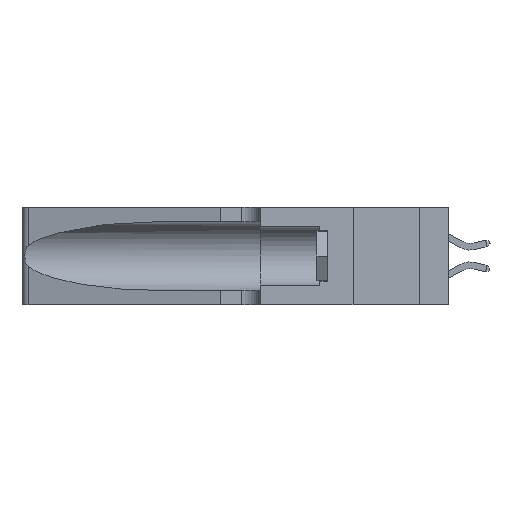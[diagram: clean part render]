
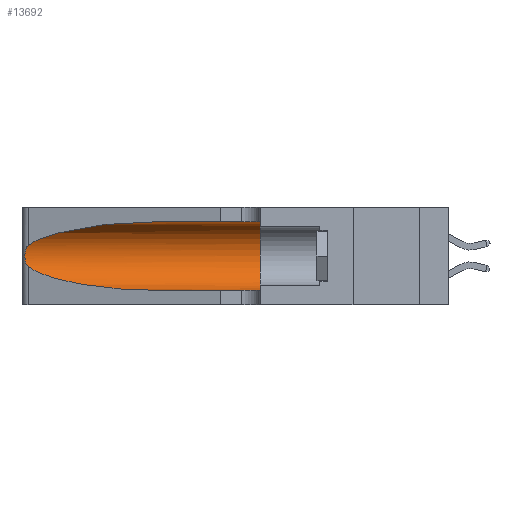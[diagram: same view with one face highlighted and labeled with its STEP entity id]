
A CAD part, left-side view. The second image highlights one B-rep face of the part: STEP entity #13692.
In plain terms, the highlighted cylindrical face has radius 3.308 mm (diameter 6.617 mm), a partial arc.
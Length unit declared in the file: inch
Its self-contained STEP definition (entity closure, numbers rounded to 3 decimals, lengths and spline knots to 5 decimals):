
#165 = FACE_OUTER_BOUND ( 'NONE', #13969, .T. ) ;
#880 = CARTESIAN_POINT ( 'NONE',  ( 0.1305, 0.72297, 0.05475 ) ) ;
#1026 = CARTESIAN_POINT ( 'NONE',  ( 0.25856, 1.23593, 0.16098 ) ) ;
#2822 = CARTESIAN_POINT ( 'NONE',  ( 0.1305, 1.61858, 0.05475 ) ) ;
#2941 = CARTESIAN_POINT ( 'NONE',  ( 0.25787, 1.23484, 0.2124 ) ) ;
#3270 = EDGE_CURVE ( 'NONE', #7609, #3434, #14867, .T. ) ;
#3434 = VERTEX_POINT ( 'NONE', #4056 ) ;
#3555 = LINE ( 'NONE', #2822, #7348 ) ;
#3957 = ORIENTED_EDGE ( 'NONE', *, *, #7733, .F. ) ;
#4056 = CARTESIAN_POINT ( 'NONE',  ( 0.25487, 1.22718, 0.22369 ) ) ;
#4150 = B_SPLINE_CURVE_WITH_KNOTS ( 'NONE', 3,
 ( #14996, #6433, #4385, #2941, #21763, #4460, #9766, #11475, #15070, #1026, #11397, #13163, #4609, #7867 ),
 .UNSPECIFIED., .F., .F.,
 ( 4, 2, 2, 2, 2, 2, 4 ),
 ( 0., 0.00027, 0.00053, 0.00107, 0.0016, 0.00187, 0.00214 ),
 .UNSPECIFIED. ) ;
#4385 = CARTESIAN_POINT ( 'NONE',  ( 0.25639, 1.23184, 0.21858 ) ) ;
#4460 = CARTESIAN_POINT ( 'NONE',  ( 0.26018, 1.23835, 0.19895 ) ) ;
#4533 = CARTESIAN_POINT ( 'NONE',  ( 0.1305, 0.72297, 0.31525 ) ) ;
#4609 = CARTESIAN_POINT ( 'NONE',  ( 0.25555, 1.22993, 0.14849 ) ) ;
#4737 = CARTESIAN_POINT ( 'NONE',  ( 0.25487, 1.22718, 0.22369 ) ) ;
#5417 = DIRECTION ( 'NONE',  ( 0., 1., 0. ) ) ;
#5689 = CARTESIAN_POINT ( 'NONE',  ( 0.1305, 1.61858, 0.31525 ) ) ;
#6272 = CARTESIAN_POINT ( 'NONE',  ( 0.1305, 0.72297, 0.31525 ) ) ;
#6433 = CARTESIAN_POINT ( 'NONE',  ( 0.25555, 1.22994, 0.2215 ) ) ;
#6752 = ORIENTED_EDGE ( 'NONE', *, *, #13815, .F. ) ;
#6821 = CARTESIAN_POINT ( 'NONE',  ( 0.1305, 0.35, 0.31525 ) ) ;
#7101 = CARTESIAN_POINT ( 'NONE',  ( 0.25487, 1.22718, 0.14631 ) ) ;
#7280 = VERTEX_POINT ( 'NONE', #6821 ) ;
#7348 = VECTOR ( 'NONE', #20287, 39.37008 ) ;
#7609 = VERTEX_POINT ( 'NONE', #4533 ) ;
#7733 = EDGE_CURVE ( 'NONE', #7280, #18139, #19593, .T. ) ;
#7867 = CARTESIAN_POINT ( 'NONE',  ( 0.25487, 1.22718, 0.14631 ) ) ;
#8226 = CARTESIAN_POINT ( 'NONE',  ( 0.2373, 1.15595, 0.28018 ) ) ;
#9071 = AXIS2_PLACEMENT_3D ( 'NONE', #10412, #5417, #20990 ) ;
#9357 = ORIENTED_EDGE ( 'NONE', *, *, #20244, .T. ) ;
#9373 = CARTESIAN_POINT ( 'NONE',  ( 0.25487, 1.22718, 0.14631 ) ) ;
#9447 = CARTESIAN_POINT ( 'NONE',  ( 0.1305, 0.72297, 0.05475 ) ) ;
#9766 = CARTESIAN_POINT ( 'NONE',  ( 0.26075, 1.23896, 0.19203 ) ) ;
#9852 =( BOUNDED_CURVE ( )  B_SPLINE_CURVE ( 3, ( #9373, #21517, #12824, #9447 ),
 .UNSPECIFIED., .F., .F. ) 
 B_SPLINE_CURVE_WITH_KNOTS ( ( 4, 4 ),
 ( 3.44316, 4.71239 ),
 .UNSPECIFIED. ) 
 CURVE ( )  GEOMETRIC_REPRESENTATION_ITEM ( )  RATIONAL_B_SPLINE_CURVE ( ( 1., 0.87, 0.87, 1. ) ) 
 REPRESENTATION_ITEM ( '' )  );
#9864 = AXIS2_PLACEMENT_3D ( 'NONE', #13708, #13776, #15459 ) ;
#10412 = CARTESIAN_POINT ( 'NONE',  ( 0.1305, 0.35, 0.185 ) ) ;
#11397 = CARTESIAN_POINT ( 'NONE',  ( 0.25789, 1.23486, 0.15765 ) ) ;
#11475 = CARTESIAN_POINT ( 'NONE',  ( 0.26075, 1.23896, 0.178 ) ) ;
#11665 = VERTEX_POINT ( 'NONE', #7101 ) ;
#12470 = DIRECTION ( 'NONE',  ( 0., -1., 0. ) ) ;
#12645 = CYLINDRICAL_SURFACE ( 'NONE', #9864, 0.13025 ) ;
#12824 = CARTESIAN_POINT ( 'NONE',  ( 0.18966, 0.96281, 0.05475 ) ) ;
#13163 = CARTESIAN_POINT ( 'NONE',  ( 0.25639, 1.23186, 0.15144 ) ) ;
#13692 = ADVANCED_FACE ( 'NONE', ( #165 ), #12645, .F. ) ;
#13708 = CARTESIAN_POINT ( 'NONE',  ( 0.1305, 1.61858, 0.185 ) ) ;
#13776 = DIRECTION ( 'NONE',  ( 0., -1., 0. ) ) ;
#13815 = EDGE_CURVE ( 'NONE', #7609, #7280, #17025, .T. ) ;
#13969 = EDGE_LOOP ( 'NONE', ( #15012, #16741, #16738, #9357, #3957, #6752 ) ) ;
#14867 =( BOUNDED_CURVE ( )  B_SPLINE_CURVE ( 3, ( #6272, #18365, #8226, #4737 ),
 .UNSPECIFIED., .F., .T. ) 
 B_SPLINE_CURVE_WITH_KNOTS ( ( 4, 4 ),
 ( 1.5708, 2.84003 ),
 .UNSPECIFIED. ) 
 CURVE ( )  GEOMETRIC_REPRESENTATION_ITEM ( )  RATIONAL_B_SPLINE_CURVE ( ( 1., 0.87, 0.87, 1. ) ) 
 REPRESENTATION_ITEM ( '' )  );
#14996 = CARTESIAN_POINT ( 'NONE',  ( 0.25487, 1.22718, 0.22369 ) ) ;
#15012 = ORIENTED_EDGE ( 'NONE', *, *, #3270, .T. ) ;
#15070 = CARTESIAN_POINT ( 'NONE',  ( 0.26017, 1.23833, 0.17102 ) ) ;
#15082 = VERTEX_POINT ( 'NONE', #880 ) ;
#15459 = DIRECTION ( 'NONE',  ( 0., 0., -1. ) ) ;
#15522 = EDGE_CURVE ( 'NONE', #3434, #11665, #4150, .T. ) ;
#16738 = ORIENTED_EDGE ( 'NONE', *, *, #21498, .T. ) ;
#16741 = ORIENTED_EDGE ( 'NONE', *, *, #15522, .T. ) ;
#17025 = LINE ( 'NONE', #5689, #17571 ) ;
#17571 = VECTOR ( 'NONE', #12470, 39.37008 ) ;
#18139 = VERTEX_POINT ( 'NONE', #19052 ) ;
#18365 = CARTESIAN_POINT ( 'NONE',  ( 0.18966, 0.96281, 0.31525 ) ) ;
#19052 = CARTESIAN_POINT ( 'NONE',  ( 0.1305, 0.35, 0.05475 ) ) ;
#19593 = CIRCLE ( 'NONE', #9071, 0.13025 ) ;
#20244 = EDGE_CURVE ( 'NONE', #15082, #18139, #3555, .T. ) ;
#20287 = DIRECTION ( 'NONE',  ( 0., -1., 0. ) ) ;
#20990 = DIRECTION ( 'NONE',  ( 0., 0., 1. ) ) ;
#21498 = EDGE_CURVE ( 'NONE', #11665, #15082, #9852, .T. ) ;
#21517 = CARTESIAN_POINT ( 'NONE',  ( 0.2373, 1.15595, 0.08982 ) ) ;
#21763 = CARTESIAN_POINT ( 'NONE',  ( 0.25854, 1.2359, 0.20912 ) ) ;
